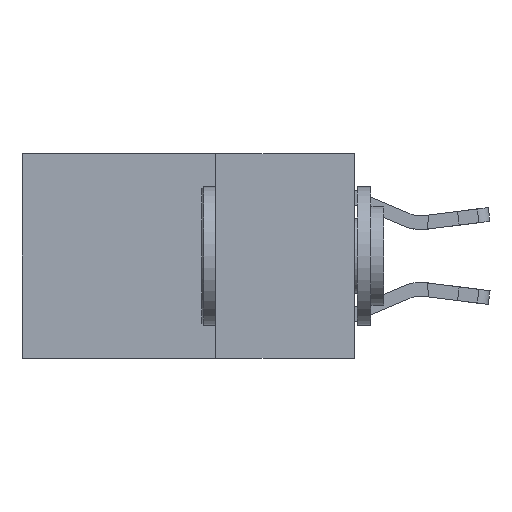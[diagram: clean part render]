
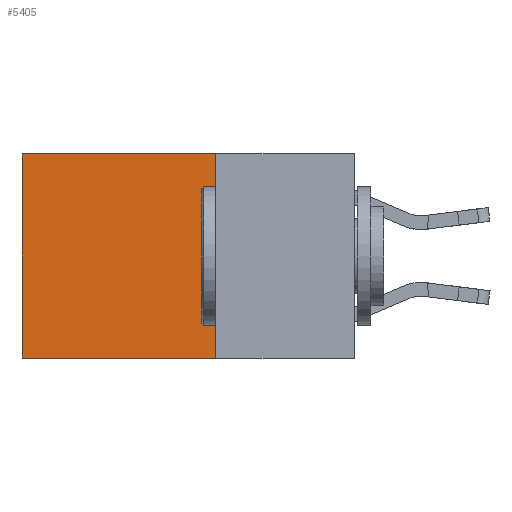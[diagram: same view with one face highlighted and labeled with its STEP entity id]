
A CAD part, left-side view. The second image highlights one B-rep face of the part: STEP entity #5405.
In plain terms, the highlighted planar face has unit normal (-1, 0, 0).
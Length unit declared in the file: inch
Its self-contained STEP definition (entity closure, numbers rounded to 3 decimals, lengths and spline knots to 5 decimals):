
#51 = DIRECTION ( 'NONE',  ( 0., 1., 0. ) ) ;
#134 = VECTOR ( 'NONE', #51, 39.37008 ) ;
#189 = VECTOR ( 'NONE', #11941, 39.37008 ) ;
#364 = DIRECTION ( 'NONE',  ( 0., 1., 0. ) ) ;
#1124 = VECTOR ( 'NONE', #364, 39.37008 ) ;
#1378 = FACE_OUTER_BOUND ( 'NONE', #1890, .T. ) ;
#1481 = CARTESIAN_POINT ( 'NONE',  ( 0.2625, 0.25, -0.37 ) ) ;
#1890 = EDGE_LOOP ( 'NONE', ( #5601, #9790, #14072, #13285 ) ) ;
#1921 = CARTESIAN_POINT ( 'NONE',  ( 0.2625, 0.25, 0. ) ) ;
#1988 = CARTESIAN_POINT ( 'NONE',  ( 0.2625, 0.25, 0. ) ) ;
#2594 = CARTESIAN_POINT ( 'NONE',  ( 0.2625, 0.6, -0.37 ) ) ;
#2898 = VERTEX_POINT ( 'NONE', #1988 ) ;
#2998 = CARTESIAN_POINT ( 'NONE',  ( 0.2625, 0.25, -0.37 ) ) ;
#4330 = VERTEX_POINT ( 'NONE', #2594 ) ;
#4787 = CARTESIAN_POINT ( 'NONE',  ( 0.2625, 0.6, 0. ) ) ;
#5405 = ADVANCED_FACE ( 'NONE', ( #1378 ), #14032, .F. ) ;
#5601 = ORIENTED_EDGE ( 'NONE', *, *, #7463, .T. ) ;
#7180 = VERTEX_POINT ( 'NONE', #1481 ) ;
#7463 = EDGE_CURVE ( 'NONE', #13723, #4330, #12747, .T. ) ;
#7485 = DIRECTION ( 'NONE',  ( 0., 0., -1. ) ) ;
#8086 = DIRECTION ( 'NONE',  ( 1., 0., 0. ) ) ;
#8804 = AXIS2_PLACEMENT_3D ( 'NONE', #10950, #8086, #18346 ) ;
#9790 = ORIENTED_EDGE ( 'NONE', *, *, #15963, .F. ) ;
#10950 = CARTESIAN_POINT ( 'NONE',  ( 0.2625, 0.25, 0. ) ) ;
#11941 = DIRECTION ( 'NONE',  ( 0., 0., -1. ) ) ;
#12124 = CARTESIAN_POINT ( 'NONE',  ( 0.2625, 0.6, 0. ) ) ;
#12747 = LINE ( 'NONE', #12124, #189 ) ;
#12955 = EDGE_CURVE ( 'NONE', #2898, #13723, #16150, .T. ) ;
#13285 = ORIENTED_EDGE ( 'NONE', *, *, #12955, .T. ) ;
#13333 = CARTESIAN_POINT ( 'NONE',  ( 0.2625, 0.25, 0. ) ) ;
#13678 = EDGE_CURVE ( 'NONE', #2898, #7180, #16132, .T. ) ;
#13723 = VERTEX_POINT ( 'NONE', #4787 ) ;
#13841 = LINE ( 'NONE', #2998, #134 ) ;
#14032 = PLANE ( 'NONE',  #8804 ) ;
#14072 = ORIENTED_EDGE ( 'NONE', *, *, #13678, .F. ) ;
#14770 = VECTOR ( 'NONE', #7485, 39.37008 ) ;
#15963 = EDGE_CURVE ( 'NONE', #7180, #4330, #13841, .T. ) ;
#16132 = LINE ( 'NONE', #1921, #14770 ) ;
#16150 = LINE ( 'NONE', #13333, #1124 ) ;
#18346 = DIRECTION ( 'NONE',  ( 0., 0., -1. ) ) ;
